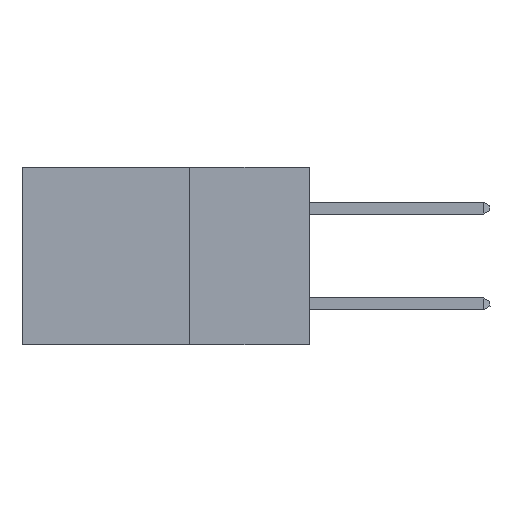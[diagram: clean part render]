
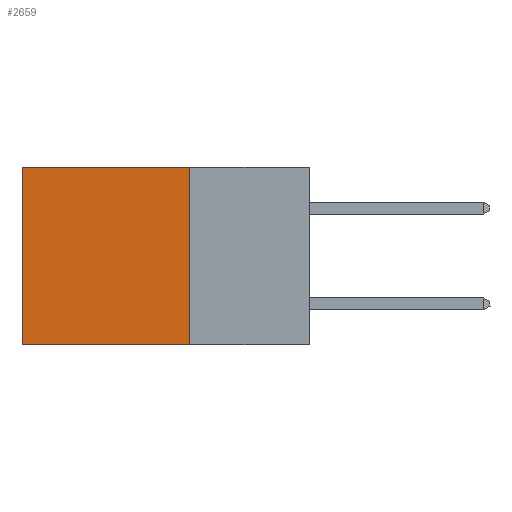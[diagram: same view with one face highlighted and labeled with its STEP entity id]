
A CAD part, left-side view. The second image highlights one B-rep face of the part: STEP entity #2659.
In plain terms, the highlighted planar face has unit normal (-1, 0, 0).
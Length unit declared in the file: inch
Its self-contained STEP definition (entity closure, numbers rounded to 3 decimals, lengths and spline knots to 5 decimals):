
#1531 = LINE ( 'NONE', #6383, #13348 ) ;
#1730 = DIRECTION ( 'NONE',  ( 0., 0., -1. ) ) ;
#2022 = DIRECTION ( 'NONE',  ( 0., 1., 0. ) ) ;
#2119 = CARTESIAN_POINT ( 'NONE',  ( 0.2875, 0.25, 0. ) ) ;
#2659 = ADVANCED_FACE ( 'NONE', ( #9545 ), #6889, .F. ) ;
#3363 = EDGE_CURVE ( 'NONE', #5542, #13003, #8219, .T. ) ;
#4698 = ORIENTED_EDGE ( 'NONE', *, *, #12626, .T. ) ;
#4911 = ORIENTED_EDGE ( 'NONE', *, *, #3363, .F. ) ;
#5362 = EDGE_LOOP ( 'NONE', ( #5589, #6023, #4911, #4698 ) ) ;
#5542 = VERTEX_POINT ( 'NONE', #10064 ) ;
#5589 = ORIENTED_EDGE ( 'NONE', *, *, #9781, .T. ) ;
#5800 = AXIS2_PLACEMENT_3D ( 'NONE', #10981, #5889, #1730 ) ;
#5889 = DIRECTION ( 'NONE',  ( 1., 0., 0. ) ) ;
#6023 = ORIENTED_EDGE ( 'NONE', *, *, #9219, .F. ) ;
#6280 = DIRECTION ( 'NONE',  ( 0., 0., -1. ) ) ;
#6383 = CARTESIAN_POINT ( 'NONE',  ( 0.2875, 0.25, -0.37 ) ) ;
#6889 = PLANE ( 'NONE',  #5800 ) ;
#7433 = DIRECTION ( 'NONE',  ( 0., 1., 0. ) ) ;
#7669 = CARTESIAN_POINT ( 'NONE',  ( 0.2875, 0.6, 0. ) ) ;
#7791 = VECTOR ( 'NONE', #2022, 39.37008 ) ;
#8219 = LINE ( 'NONE', #10496, #9182 ) ;
#8490 = LINE ( 'NONE', #7669, #11377 ) ;
#9182 = VECTOR ( 'NONE', #6280, 39.37008 ) ;
#9206 = VERTEX_POINT ( 'NONE', #12568 ) ;
#9219 = EDGE_CURVE ( 'NONE', #13003, #11211, #1531, .T. ) ;
#9545 = FACE_OUTER_BOUND ( 'NONE', #5362, .T. ) ;
#9701 = LINE ( 'NONE', #2119, #7791 ) ;
#9781 = EDGE_CURVE ( 'NONE', #9206, #11211, #8490, .T. ) ;
#10064 = CARTESIAN_POINT ( 'NONE',  ( 0.2875, 0.25, 0. ) ) ;
#10496 = CARTESIAN_POINT ( 'NONE',  ( 0.2875, 0.25, 0. ) ) ;
#10782 = CARTESIAN_POINT ( 'NONE',  ( 0.2875, 0.25, -0.37 ) ) ;
#10981 = CARTESIAN_POINT ( 'NONE',  ( 0.2875, 0.25, 0. ) ) ;
#11035 = CARTESIAN_POINT ( 'NONE',  ( 0.2875, 0.6, -0.37 ) ) ;
#11211 = VERTEX_POINT ( 'NONE', #11035 ) ;
#11377 = VECTOR ( 'NONE', #12768, 39.37008 ) ;
#12568 = CARTESIAN_POINT ( 'NONE',  ( 0.2875, 0.6, 0. ) ) ;
#12626 = EDGE_CURVE ( 'NONE', #5542, #9206, #9701, .T. ) ;
#12768 = DIRECTION ( 'NONE',  ( 0., 0., -1. ) ) ;
#13003 = VERTEX_POINT ( 'NONE', #10782 ) ;
#13348 = VECTOR ( 'NONE', #7433, 39.37008 ) ;
